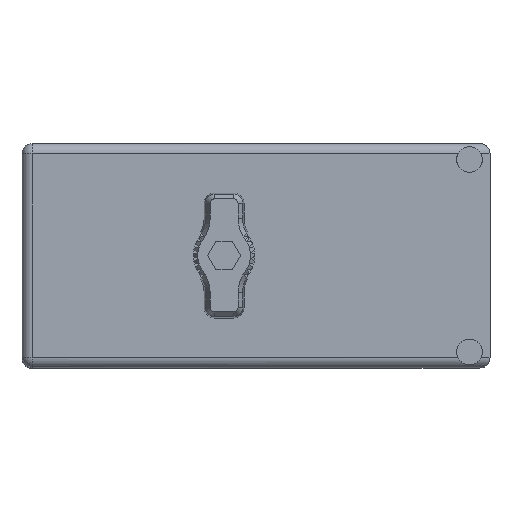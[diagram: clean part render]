
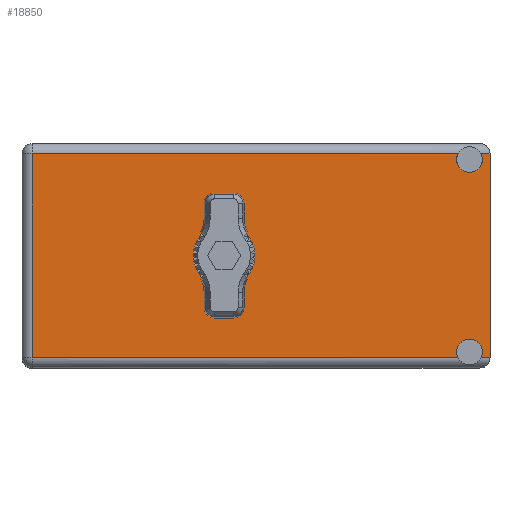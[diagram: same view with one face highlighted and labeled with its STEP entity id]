
A CAD part, top view. The second image highlights one B-rep face of the part: STEP entity #18850.
In plain terms, the highlighted face is planar.
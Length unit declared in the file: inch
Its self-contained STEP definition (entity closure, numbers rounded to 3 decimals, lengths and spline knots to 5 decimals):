
#201 = DIRECTION ( 'NONE',  ( 0., 0., 1. ) ) ;
#1172 = DIRECTION ( 'NONE',  ( 0., 1., 0. ) ) ;
#1200 = VECTOR ( 'NONE', #13693, 39.37008 ) ;
#3026 = AXIS2_PLACEMENT_3D ( 'NONE', #48717, #1172, #9815 ) ;
#3640 = CARTESIAN_POINT ( 'NONE',  ( 0., 2.03, -1.46 ) ) ;
#4929 = VERTEX_POINT ( 'NONE', #45992 ) ;
#5000 = CARTESIAN_POINT ( 'NONE',  ( 1.3775, 2.03, -0.595 ) ) ;
#5583 = EDGE_CURVE ( 'NONE', #14418, #86455, #37604, .T. ) ;
#6122 = LINE ( 'NONE', #3640, #58335 ) ;
#6366 = DIRECTION ( 'NONE',  ( 0., 1., 0. ) ) ;
#6902 = VECTOR ( 'NONE', #8192, 39.37008 ) ;
#7677 = VERTEX_POINT ( 'NONE', #8554 ) ;
#8192 = DIRECTION ( 'NONE',  ( 0., 0., 1. ) ) ;
#8410 = EDGE_CURVE ( 'NONE', #76145, #80918, #78161, .T. ) ;
#8554 = CARTESIAN_POINT ( 'NONE',  ( 1.3775, 2.03, -0.935 ) ) ;
#9000 = AXIS2_PLACEMENT_3D ( 'NONE', #43819, #29544, #9378 ) ;
#9378 = DIRECTION ( 'NONE',  ( 0., 0., 1. ) ) ;
#9815 = DIRECTION ( 'NONE',  ( 0., 0., 1. ) ) ;
#9935 = ORIENTED_EDGE ( 'NONE', *, *, #5583, .T. ) ;
#11125 = EDGE_CURVE ( 'NONE', #31967, #85462, #12222, .T. ) ;
#12222 = CIRCLE ( 'NONE', #9000, 0.0875 ) ;
#13103 = EDGE_CURVE ( 'NONE', #13601, #86455, #51707, .T. ) ;
#13601 = VERTEX_POINT ( 'NONE', #65674 ) ;
#13693 = DIRECTION ( 'NONE',  ( 1., 0., 0. ) ) ;
#14032 = VECTOR ( 'NONE', #37666, 39.37008 ) ;
#14418 = VERTEX_POINT ( 'NONE', #19083 ) ;
#15185 = CARTESIAN_POINT ( 'NONE',  ( 3.19, 2.03, -0.07 ) ) ;
#16374 = CIRCLE ( 'NONE', #27634, 0.0875 ) ;
#18144 = VERTEX_POINT ( 'NONE', #46899 ) ;
#18373 = DIRECTION ( 'NONE',  ( -1., 0., 0. ) ) ;
#18850 = ADVANCED_FACE ( 'NONE', ( #49563, #42062 ), #72292, .T. ) ;
#19083 = CARTESIAN_POINT ( 'NONE',  ( 0.07, 2.03, -0.07 ) ) ;
#19283 = EDGE_LOOP ( 'NONE', ( #9935, #84445, #51999, #55861, #70194, #84548, #45924, #47115, #74781, #19631 ) ) ;
#19631 = ORIENTED_EDGE ( 'NONE', *, *, #78887, .T. ) ;
#20236 = ORIENTED_EDGE ( 'NONE', *, *, #60061, .F. ) ;
#20355 = AXIS2_PLACEMENT_3D ( 'NONE', #45589, #6366, #31309 ) ;
#21888 = CIRCLE ( 'NONE', #3026, 0.17 ) ;
#23888 = EDGE_CURVE ( 'NONE', #76145, #13601, #61387, .T. ) ;
#27634 = AXIS2_PLACEMENT_3D ( 'NONE', #79750, #87666, #102192 ) ;
#29544 = DIRECTION ( 'NONE',  ( 0., 1., 0. ) ) ;
#31309 = DIRECTION ( 'NONE',  ( 0., 0., 1. ) ) ;
#31967 = VERTEX_POINT ( 'NONE', #63191 ) ;
#32308 = CARTESIAN_POINT ( 'NONE',  ( 0., 2.03, -1.53 ) ) ;
#35300 = CARTESIAN_POINT ( 'NONE',  ( 2.97167, 2.03, -0.07 ) ) ;
#35332 = AXIS2_PLACEMENT_3D ( 'NONE', #78107, #38847, #63518 ) ;
#35758 = AXIS2_PLACEMENT_3D ( 'NONE', #73793, #81753, #89646 ) ;
#36200 = CARTESIAN_POINT ( 'NONE',  ( 3.12833, 2.03, -1.46 ) ) ;
#36290 = CARTESIAN_POINT ( 'NONE',  ( 3.12833, 2.03, -0.07 ) ) ;
#37323 = CARTESIAN_POINT ( 'NONE',  ( 3.19, 2.03, -0.07 ) ) ;
#37604 = LINE ( 'NONE', #37323, #14032 ) ;
#37666 = DIRECTION ( 'NONE',  ( 1., 0., 0. ) ) ;
#37778 = EDGE_CURVE ( 'NONE', #18144, #31967, #16374, .T. ) ;
#38847 = DIRECTION ( 'NONE',  ( 0., 1., 0. ) ) ;
#40016 = LINE ( 'NONE', #92094, #66149 ) ;
#40157 = VERTEX_POINT ( 'NONE', #92736 ) ;
#40842 = ORIENTED_EDGE ( 'NONE', *, *, #47485, .F. ) ;
#42062 = FACE_OUTER_BOUND ( 'NONE', #19283, .T. ) ;
#43819 = CARTESIAN_POINT ( 'NONE',  ( 3.05, 2.03, -1.421 ) ) ;
#45589 = CARTESIAN_POINT ( 'NONE',  ( 1.3775, 2.03, -0.765 ) ) ;
#45924 = ORIENTED_EDGE ( 'NONE', *, *, #11125, .F. ) ;
#45992 = CARTESIAN_POINT ( 'NONE',  ( 0.07, 2.03, -1.46 ) ) ;
#46899 = CARTESIAN_POINT ( 'NONE',  ( 2.97167, 2.03, -1.46 ) ) ;
#47115 = ORIENTED_EDGE ( 'NONE', *, *, #37778, .F. ) ;
#47485 = EDGE_CURVE ( 'NONE', #51889, #7677, #21888, .T. ) ;
#48717 = CARTESIAN_POINT ( 'NONE',  ( 1.3775, 2.03, -0.765 ) ) ;
#49563 = FACE_BOUND ( 'NONE', #102883, .T. ) ;
#49957 = CARTESIAN_POINT ( 'NONE',  ( 0., 2.03, -1.46 ) ) ;
#50408 = CIRCLE ( 'NONE', #20355, 0.17 ) ;
#51707 = CIRCLE ( 'NONE', #35758, 0.0875 ) ;
#51889 = VERTEX_POINT ( 'NONE', #5000 ) ;
#51999 = ORIENTED_EDGE ( 'NONE', *, *, #23888, .F. ) ;
#55861 = ORIENTED_EDGE ( 'NONE', *, *, #8410, .T. ) ;
#56656 = DIRECTION ( 'NONE',  ( 0., 1., 0. ) ) ;
#58335 = VECTOR ( 'NONE', #59177, 39.37008 ) ;
#59177 = DIRECTION ( 'NONE',  ( -1., 0., 0. ) ) ;
#60061 = EDGE_CURVE ( 'NONE', #7677, #51889, #50408, .T. ) ;
#61387 = CIRCLE ( 'NONE', #35332, 0.0875 ) ;
#63191 = CARTESIAN_POINT ( 'NONE',  ( 3.05, 2.03, -1.3335 ) ) ;
#63518 = DIRECTION ( 'NONE',  ( 0., 0., 1. ) ) ;
#65674 = CARTESIAN_POINT ( 'NONE',  ( 3.05, 2.03, -0.1965 ) ) ;
#66149 = VECTOR ( 'NONE', #201, 39.37008 ) ;
#68889 = CARTESIAN_POINT ( 'NONE',  ( 3.19, 2.03, -0.07 ) ) ;
#70194 = ORIENTED_EDGE ( 'NONE', *, *, #87388, .F. ) ;
#72292 = PLANE ( 'NONE',  #102030 ) ;
#73373 = EDGE_CURVE ( 'NONE', #40157, #85462, #6122, .T. ) ;
#73793 = CARTESIAN_POINT ( 'NONE',  ( 3.05, 2.03, -0.109 ) ) ;
#74258 = VECTOR ( 'NONE', #18373, 39.37008 ) ;
#74781 = ORIENTED_EDGE ( 'NONE', *, *, #82387, .T. ) ;
#76145 = VERTEX_POINT ( 'NONE', #36290 ) ;
#78107 = CARTESIAN_POINT ( 'NONE',  ( 3.05, 2.03, -0.109 ) ) ;
#78161 = LINE ( 'NONE', #68889, #1200 ) ;
#78887 = EDGE_CURVE ( 'NONE', #4929, #14418, #40016, .T. ) ;
#79750 = CARTESIAN_POINT ( 'NONE',  ( 3.05, 2.03, -1.421 ) ) ;
#80918 = VERTEX_POINT ( 'NONE', #15185 ) ;
#81753 = DIRECTION ( 'NONE',  ( 0., 1., 0. ) ) ;
#82201 = CARTESIAN_POINT ( 'NONE',  ( 3.19, 2.03, 0. ) ) ;
#82387 = EDGE_CURVE ( 'NONE', #18144, #4929, #102722, .T. ) ;
#84445 = ORIENTED_EDGE ( 'NONE', *, *, #13103, .F. ) ;
#84548 = ORIENTED_EDGE ( 'NONE', *, *, #73373, .T. ) ;
#85462 = VERTEX_POINT ( 'NONE', #36200 ) ;
#86455 = VERTEX_POINT ( 'NONE', #35300 ) ;
#87388 = EDGE_CURVE ( 'NONE', #40157, #80918, #99893, .T. ) ;
#87666 = DIRECTION ( 'NONE',  ( 0., 1., 0. ) ) ;
#88520 = DIRECTION ( 'NONE',  ( 0., 0., 1. ) ) ;
#89646 = DIRECTION ( 'NONE',  ( 0., 0., 1. ) ) ;
#92094 = CARTESIAN_POINT ( 'NONE',  ( 0.07, 2.03, -1.53 ) ) ;
#92736 = CARTESIAN_POINT ( 'NONE',  ( 3.19, 2.03, -1.46 ) ) ;
#99893 = LINE ( 'NONE', #82201, #6902 ) ;
#102030 = AXIS2_PLACEMENT_3D ( 'NONE', #32308, #56656, #88520 ) ;
#102192 = DIRECTION ( 'NONE',  ( 0., 0., 1. ) ) ;
#102722 = LINE ( 'NONE', #49957, #74258 ) ;
#102883 = EDGE_LOOP ( 'NONE', ( #40842, #20236 ) ) ;
